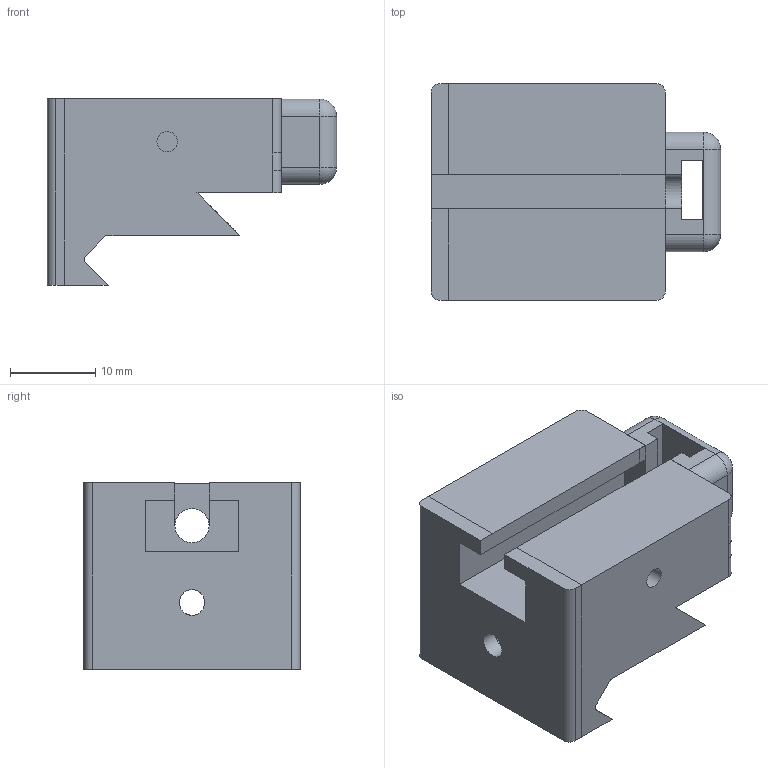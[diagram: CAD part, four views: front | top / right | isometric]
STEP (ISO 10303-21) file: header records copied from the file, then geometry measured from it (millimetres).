
FILE_DESCRIPTION(('FreeCAD Model'),'2;1');
FILE_NAME('sight base screw adjust.step','2018-04-06T19:14:14',('Author'),(''), 'Open CASCADE STEP processor 6.8','FreeCAD','Unknown');
FILE_SCHEMA(('AUTOMOTIVE_DESIGN_CC2 { 1 2 10303 214 -1 1 5 4 }'));
Length unit declared in the file: millimetre
Products named in the file (1): Fillet001
Bounding box: 33.9 x 25.4 x 21.86 mm (x, y, z)
Volume: 9422.7 mm3; surface area: 5004.5 mm2
Topology: 1 solids, 1 shells, 69 faces, 188 edges, 117 vertices
Faces by surface type: plane 43, cylinder 22, sphere 4
Full cylindrical faces by diameter (mm): 2.4 x1, 2.99 x1, 3 x1, 4 x1
Entity records: 4667 total; most frequent: CARTESIAN_POINT 1056, DIRECTION 639, LINE 398, VECTOR 398, ORIENTED_EDGE 368, PCURVE 368, DEFINITIONAL_REPRESENTATION 368, EDGE_CURVE 184
